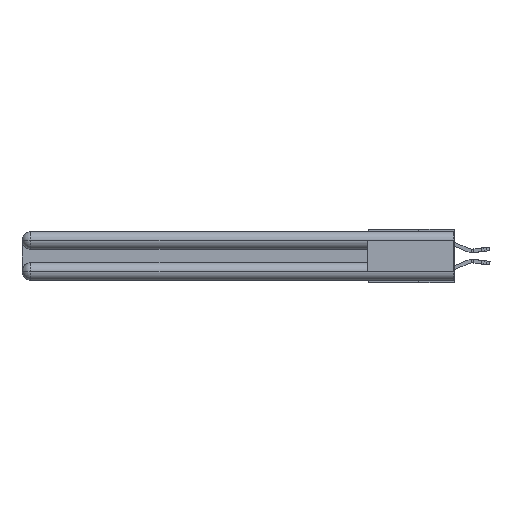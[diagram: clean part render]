
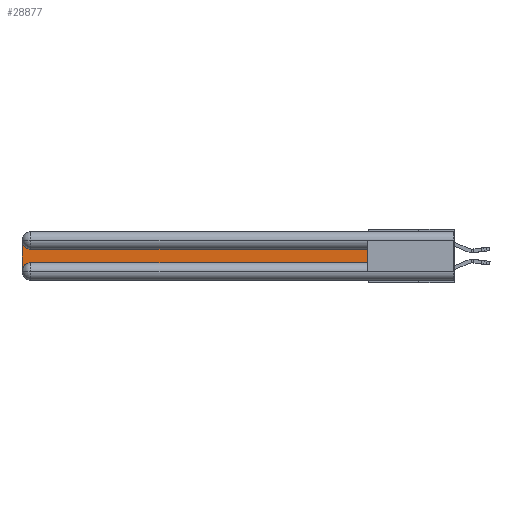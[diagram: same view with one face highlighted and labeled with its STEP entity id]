
A CAD part, left-side view. The second image highlights one B-rep face of the part: STEP entity #28877.
In plain terms, the highlighted planar face has unit normal (-1, 0, 0).
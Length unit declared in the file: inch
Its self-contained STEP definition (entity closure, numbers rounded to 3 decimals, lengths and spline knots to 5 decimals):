
#306 = ORIENTED_EDGE ( 'NONE', *, *, #12834, .T. ) ;
#827 = CARTESIAN_POINT ( 'NONE',  ( 0.075, 2.94, -0.1225 ) ) ;
#1339 = DIRECTION ( 'NONE',  ( 1., 0., 0. ) ) ;
#1897 = VECTOR ( 'NONE', #15927, 39.37008 ) ;
#2104 = DIRECTION ( 'NONE',  ( 0., 0., 1. ) ) ;
#2606 = EDGE_LOOP ( 'NONE', ( #306, #17447, #6903, #21544, #23445, #8835 ) ) ;
#3268 = AXIS2_PLACEMENT_3D ( 'NONE', #7997, #1339, #12820 ) ;
#3990 = CIRCLE ( 'NONE', #9324, 0.06 ) ;
#5266 = CIRCLE ( 'NONE', #20221, 0.06 ) ;
#5431 = CARTESIAN_POINT ( 'NONE',  ( 0.075, 3., -0.2175 ) ) ;
#5842 = PLANE ( 'NONE',  #3268 ) ;
#5919 = CARTESIAN_POINT ( 'NONE',  ( 0.075, 3., -0.0625 ) ) ;
#6061 = DIRECTION ( 'NONE',  ( 0., -1., 0. ) ) ;
#6165 = CARTESIAN_POINT ( 'NONE',  ( 0.075, 0.6, -0.2175 ) ) ;
#6903 = ORIENTED_EDGE ( 'NONE', *, *, #22004, .T. ) ;
#7009 = DIRECTION ( 'NONE',  ( 0., 0., -1. ) ) ;
#7322 = DIRECTION ( 'NONE',  ( 1., 0., 0. ) ) ;
#7630 = EDGE_CURVE ( 'NONE', #18455, #12616, #21876, .T. ) ;
#7997 = CARTESIAN_POINT ( 'NONE',  ( 0.075, 3., -0.1225 ) ) ;
#8835 = ORIENTED_EDGE ( 'NONE', *, *, #12841, .T. ) ;
#9324 = AXIS2_PLACEMENT_3D ( 'NONE', #13372, #26941, #15391 ) ;
#9364 = CARTESIAN_POINT ( 'NONE',  ( 0.075, 2.94, -0.0625 ) ) ;
#9784 = CARTESIAN_POINT ( 'NONE',  ( 0.075, 0.6, -0.2175 ) ) ;
#10223 = LINE ( 'NONE', #9784, #24534 ) ;
#10825 = VERTEX_POINT ( 'NONE', #15399 ) ;
#11555 = CARTESIAN_POINT ( 'NONE',  ( 0.075, 2.94, -0.2175 ) ) ;
#11826 = CARTESIAN_POINT ( 'NONE',  ( 0.075, 3., -0.2775 ) ) ;
#12616 = VERTEX_POINT ( 'NONE', #6165 ) ;
#12820 = DIRECTION ( 'NONE',  ( 0., 0., -1. ) ) ;
#12834 = EDGE_CURVE ( 'NONE', #10825, #28610, #13108, .T. ) ;
#12841 = EDGE_CURVE ( 'NONE', #12616, #10825, #10223, .T. ) ;
#13108 = LINE ( 'NONE', #21207, #1897 ) ;
#13268 = VECTOR ( 'NONE', #14940, 39.37008 ) ;
#13372 = CARTESIAN_POINT ( 'NONE',  ( 0.075, 2.94, -0.2775 ) ) ;
#14940 = DIRECTION ( 'NONE',  ( 0., 0., -1. ) ) ;
#15391 = DIRECTION ( 'NONE',  ( 0., 0., -1. ) ) ;
#15399 = CARTESIAN_POINT ( 'NONE',  ( 0.075, 0.6, -0.1225 ) ) ;
#15927 = DIRECTION ( 'NONE',  ( 0., 1., 0. ) ) ;
#16019 = EDGE_CURVE ( 'NONE', #28610, #19896, #5266, .T. ) ;
#17447 = ORIENTED_EDGE ( 'NONE', *, *, #16019, .T. ) ;
#17790 = CARTESIAN_POINT ( 'NONE',  ( 0.075, 0.6, -0.2175 ) ) ;
#18301 = LINE ( 'NONE', #5431, #13268 ) ;
#18455 = VERTEX_POINT ( 'NONE', #11555 ) ;
#18687 = VECTOR ( 'NONE', #6061, 39.37008 ) ;
#19896 = VERTEX_POINT ( 'NONE', #5919 ) ;
#20221 = AXIS2_PLACEMENT_3D ( 'NONE', #9364, #7322, #7009 ) ;
#20376 = EDGE_CURVE ( 'NONE', #23678, #18455, #3990, .T. ) ;
#21207 = CARTESIAN_POINT ( 'NONE',  ( 0.075, 0.6, -0.1225 ) ) ;
#21544 = ORIENTED_EDGE ( 'NONE', *, *, #20376, .T. ) ;
#21876 = LINE ( 'NONE', #17790, #18687 ) ;
#22004 = EDGE_CURVE ( 'NONE', #19896, #23678, #18301, .T. ) ;
#23445 = ORIENTED_EDGE ( 'NONE', *, *, #7630, .T. ) ;
#23678 = VERTEX_POINT ( 'NONE', #11826 ) ;
#24534 = VECTOR ( 'NONE', #2104, 39.37008 ) ;
#26941 = DIRECTION ( 'NONE',  ( 1., 0., 0. ) ) ;
#28610 = VERTEX_POINT ( 'NONE', #827 ) ;
#28877 = ADVANCED_FACE ( 'NONE', ( #29614 ), #5842, .F. ) ;
#29614 = FACE_OUTER_BOUND ( 'NONE', #2606, .T. ) ;
